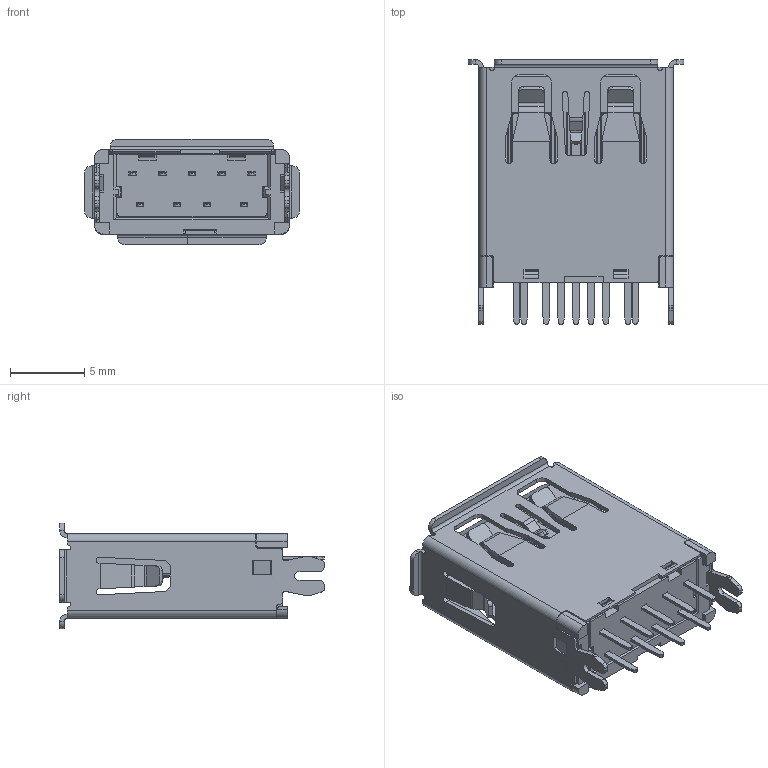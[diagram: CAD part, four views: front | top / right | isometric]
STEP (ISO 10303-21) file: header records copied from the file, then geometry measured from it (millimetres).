
FILE_DESCRIPTION (( 'STEP AP214' ), '1' );
FILE_NAME ('690F109-64C-012.STEP', '2021-01-14T18:10:06', ( '' ), ( '' ), 'SwSTEP 2.0', 'SolidWorks 2020', '' );
FILE_SCHEMA (( 'AUTOMOTIVE_DESIGN' ));
Length unit declared in the file: millimetre
Products named in the file (6): Insulator1 690F109-64C-012; Insulator2 690F109-64C-012; Contact 2.0 690F109-64C-012; Contact 3.0 690F109-64C-012; 690F109-64C-012; Shell 690F109-64C-012
Assembly tree (12 placements, depth 2):
  690F109-64C-012
    Insulator1 690F109-64C-012
    Contact 3.0 690F109-64C-012  x5
    Contact 2.0 690F109-64C-012  x4
    Insulator2 690F109-64C-012
    Shell 690F109-64C-012
Bounding box: 14.5 x 17.8 x 7.12 mm (x, y, z)
Volume: 522.4 mm3; surface area: 2611.5 mm2
Topology: 12 solids, 12 shells, 2136 faces, 6080 edges, 3923 vertices
Faces by surface type: plane 1377, cylinder 635, bspline 92, cone 32
Entity records: 47027 total; most frequent: CARTESIAN_POINT 9348, ORIENTED_EDGE 8126, DIRECTION 7445, EDGE_CURVE 4063, LINE 3269, VECTOR 3269, VERTEX_POINT 2609, AXIS2_PLACEMENT_3D 2088
